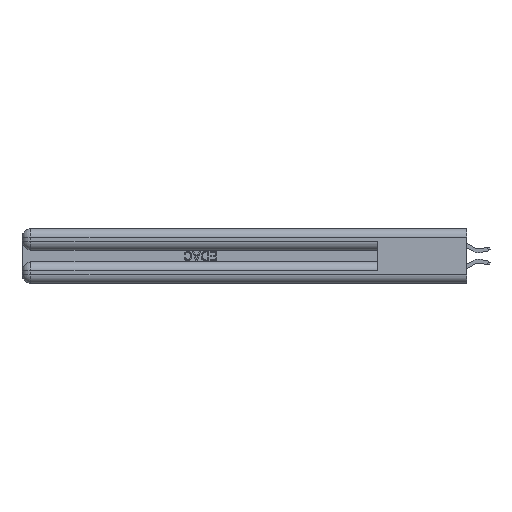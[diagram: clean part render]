
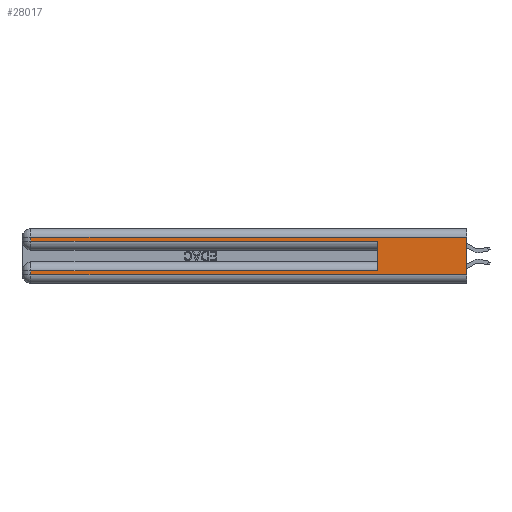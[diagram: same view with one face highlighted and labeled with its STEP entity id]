
A CAD part, left-side view. The second image highlights one B-rep face of the part: STEP entity #28017.
In plain terms, the highlighted planar face has unit normal (-1, 0, 0).
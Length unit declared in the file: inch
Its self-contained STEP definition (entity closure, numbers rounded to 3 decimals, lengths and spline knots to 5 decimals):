
#671 = EDGE_LOOP ( 'NONE', ( #35292, #15479, #45693, #27764, #27259, #16987, #31607, #35919 ) ) ;
#961 = CARTESIAN_POINT ( 'NONE',  ( 0., 0., 0.06 ) ) ;
#1723 = DIRECTION ( 'NONE',  ( 0., 1., 0. ) ) ;
#2850 = CARTESIAN_POINT ( 'NONE',  ( 0., 2.94, 0.085 ) ) ;
#3684 = VECTOR ( 'NONE', #22905, 39.37008 ) ;
#8356 = CARTESIAN_POINT ( 'NONE',  ( 0., 2.94, 0.31 ) ) ;
#10579 = CARTESIAN_POINT ( 'NONE',  ( 0., 0., 0.31 ) ) ;
#11126 = VECTOR ( 'NONE', #43837, 39.37008 ) ;
#11238 = CARTESIAN_POINT ( 'NONE',  ( 0., 0., 0.37 ) ) ;
#12853 = DIRECTION ( 'NONE',  ( 0., 0., -1. ) ) ;
#12950 = EDGE_CURVE ( 'NONE', #33452, #37326, #40000, .T. ) ;
#13283 = VERTEX_POINT ( 'NONE', #2850 ) ;
#14882 = DIRECTION ( 'NONE',  ( 1., 0., 0. ) ) ;
#15479 = ORIENTED_EDGE ( 'NONE', *, *, #24218, .T. ) ;
#16113 = CARTESIAN_POINT ( 'NONE',  ( 0., 0., 0.31 ) ) ;
#16367 = VERTEX_POINT ( 'NONE', #10579 ) ;
#16987 = ORIENTED_EDGE ( 'NONE', *, *, #46774, .T. ) ;
#17464 = VERTEX_POINT ( 'NONE', #961 ) ;
#18199 = DIRECTION ( 'NONE',  ( 0., 0., -1. ) ) ;
#18961 = CARTESIAN_POINT ( 'NONE',  ( 0., 0.6, 0.085 ) ) ;
#19434 = VECTOR ( 'NONE', #1723, 39.37008 ) ;
#19738 = LINE ( 'NONE', #30917, #28243 ) ;
#21171 = DIRECTION ( 'NONE',  ( 0., -1., 0. ) ) ;
#21475 = VECTOR ( 'NONE', #24422, 39.37008 ) ;
#21479 = EDGE_CURVE ( 'NONE', #13283, #33531, #32266, .T. ) ;
#22371 = VECTOR ( 'NONE', #21171, 39.37008 ) ;
#22905 = DIRECTION ( 'NONE',  ( 0., 1., 0. ) ) ;
#23419 = VERTEX_POINT ( 'NONE', #26499 ) ;
#23826 = VECTOR ( 'NONE', #18199, 39.37008 ) ;
#24218 = EDGE_CURVE ( 'NONE', #16367, #37160, #29077, .T. ) ;
#24422 = DIRECTION ( 'NONE',  ( 0., 0., -1. ) ) ;
#25864 = CARTESIAN_POINT ( 'NONE',  ( 0., 0.6, 0.145 ) ) ;
#25945 = EDGE_CURVE ( 'NONE', #16367, #17464, #33444, .T. ) ;
#26499 = CARTESIAN_POINT ( 'NONE',  ( 0., 2.94, 0.285 ) ) ;
#26861 = CARTESIAN_POINT ( 'NONE',  ( 0., 2.94, 0.06 ) ) ;
#27259 = ORIENTED_EDGE ( 'NONE', *, *, #12950, .F. ) ;
#27764 = ORIENTED_EDGE ( 'NONE', *, *, #35019, .T. ) ;
#28017 = ADVANCED_FACE ( 'NONE', ( #40633 ), #32961, .F. ) ;
#28243 = VECTOR ( 'NONE', #12853, 39.37008 ) ;
#29077 = LINE ( 'NONE', #16113, #19434 ) ;
#30917 = CARTESIAN_POINT ( 'NONE',  ( 0., 2.94, 0.37 ) ) ;
#31526 = CARTESIAN_POINT ( 'NONE',  ( 0., 2.94, 0.37 ) ) ;
#31607 = ORIENTED_EDGE ( 'NONE', *, *, #21479, .T. ) ;
#31920 = EDGE_CURVE ( 'NONE', #37160, #23419, #19738, .T. ) ;
#32266 = LINE ( 'NONE', #31526, #21475 ) ;
#32315 = CARTESIAN_POINT ( 'NONE',  ( 0., 0., 0.37 ) ) ;
#32961 = PLANE ( 'NONE',  #40934 ) ;
#33444 = LINE ( 'NONE', #32315, #23826 ) ;
#33452 = VERTEX_POINT ( 'NONE', #18961 ) ;
#33531 = VERTEX_POINT ( 'NONE', #26861 ) ;
#33766 = LINE ( 'NONE', #40907, #3684 ) ;
#35019 = EDGE_CURVE ( 'NONE', #23419, #37326, #42714, .T. ) ;
#35292 = ORIENTED_EDGE ( 'NONE', *, *, #25945, .F. ) ;
#35919 = ORIENTED_EDGE ( 'NONE', *, *, #40683, .T. ) ;
#37160 = VERTEX_POINT ( 'NONE', #8356 ) ;
#37326 = VERTEX_POINT ( 'NONE', #38297 ) ;
#38297 = CARTESIAN_POINT ( 'NONE',  ( 0., 0.6, 0.285 ) ) ;
#39197 = CARTESIAN_POINT ( 'NONE',  ( 0., 0., 0.285 ) ) ;
#40000 = LINE ( 'NONE', #25864, #11126 ) ;
#40197 = DIRECTION ( 'NONE',  ( 0., 0., -1. ) ) ;
#40633 = FACE_OUTER_BOUND ( 'NONE', #671, .T. ) ;
#40683 = EDGE_CURVE ( 'NONE', #33531, #17464, #44019, .T. ) ;
#40907 = CARTESIAN_POINT ( 'NONE',  ( 0., 0., 0.085 ) ) ;
#40934 = AXIS2_PLACEMENT_3D ( 'NONE', #11238, #14882, #40197 ) ;
#42586 = CARTESIAN_POINT ( 'NONE',  ( 0., 0., 0.06 ) ) ;
#42714 = LINE ( 'NONE', #39197, #22371 ) ;
#42895 = VECTOR ( 'NONE', #46168, 39.37008 ) ;
#43837 = DIRECTION ( 'NONE',  ( 0., 0., 1. ) ) ;
#44019 = LINE ( 'NONE', #42586, #42895 ) ;
#45693 = ORIENTED_EDGE ( 'NONE', *, *, #31920, .T. ) ;
#46168 = DIRECTION ( 'NONE',  ( 0., -1., 0. ) ) ;
#46774 = EDGE_CURVE ( 'NONE', #33452, #13283, #33766, .T. ) ;
